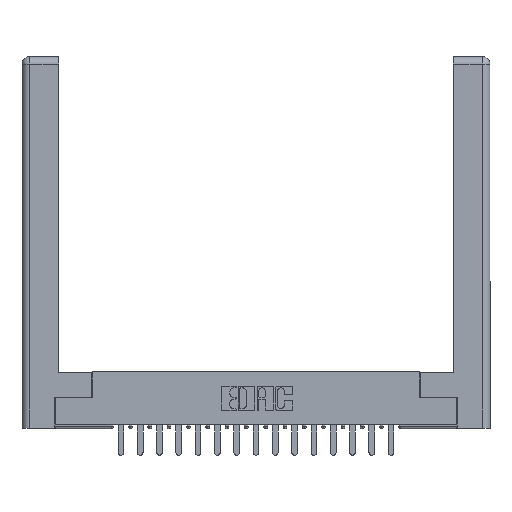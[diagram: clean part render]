
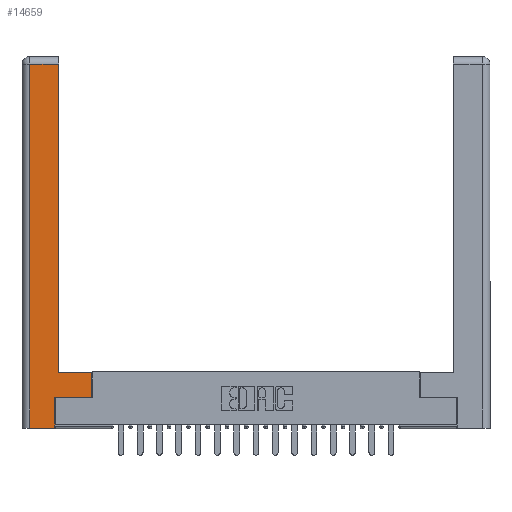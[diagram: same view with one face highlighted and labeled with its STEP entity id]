
A CAD part, top view. The second image highlights one B-rep face of the part: STEP entity #14659.
In plain terms, the highlighted planar face has unit normal (0, 0, 1).
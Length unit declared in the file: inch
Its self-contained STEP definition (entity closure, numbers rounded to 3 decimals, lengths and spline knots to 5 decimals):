
#138 = LINE ( 'NONE', #17752, #3976 ) ;
#511 = EDGE_CURVE ( 'NONE', #17838, #16991, #8730, .T. ) ;
#798 = ORIENTED_EDGE ( 'NONE', *, *, #15813, .T. ) ;
#850 = LINE ( 'NONE', #16740, #11092 ) ;
#1179 = CARTESIAN_POINT ( 'NONE',  ( 0.265, 0.245, 0. ) ) ;
#1506 = CARTESIAN_POINT ( 'NONE',  ( 0.0615, 2.94, 0. ) ) ;
#2007 = CARTESIAN_POINT ( 'NONE',  ( 0.0615, 2.94, 0. ) ) ;
#2164 = ORIENTED_EDGE ( 'NONE', *, *, #18892, .T. ) ;
#2183 = DIRECTION ( 'NONE',  ( 1., 0., 0. ) ) ;
#2369 = VECTOR ( 'NONE', #8172, 39.37008 ) ;
#2411 = FACE_OUTER_BOUND ( 'NONE', #13068, .T. ) ;
#2498 = EDGE_CURVE ( 'NONE', #12459, #17838, #14176, .T. ) ;
#2706 = PLANE ( 'NONE',  #8961 ) ;
#3361 = CARTESIAN_POINT ( 'NONE',  ( 0.565, 0.245, 0. ) ) ;
#3501 = VERTEX_POINT ( 'NONE', #12712 ) ;
#3976 = VECTOR ( 'NONE', #19290, 39.37008 ) ;
#4780 = CARTESIAN_POINT ( 'NONE',  ( 0.295, 0.45, 0. ) ) ;
#5429 = CARTESIAN_POINT ( 'NONE',  ( 0.295, 2.94, 0. ) ) ;
#5454 = ORIENTED_EDGE ( 'NONE', *, *, #511, .T. ) ;
#5558 = LINE ( 'NONE', #10978, #12875 ) ;
#5668 = EDGE_CURVE ( 'NONE', #6806, #17749, #12123, .T. ) ;
#6457 = DIRECTION ( 'NONE',  ( 0., -1., 0. ) ) ;
#6792 = DIRECTION ( 'NONE',  ( -1., 0., 0. ) ) ;
#6806 = VERTEX_POINT ( 'NONE', #5429 ) ;
#7336 = EDGE_CURVE ( 'NONE', #16514, #3501, #850, .T. ) ;
#7434 = DIRECTION ( 'NONE',  ( 0., 1., 0. ) ) ;
#8172 = DIRECTION ( 'NONE',  ( 0., 1., 0. ) ) ;
#8730 = LINE ( 'NONE', #9807, #2369 ) ;
#8961 = AXIS2_PLACEMENT_3D ( 'NONE', #15368, #13759, #16874 ) ;
#9242 = CARTESIAN_POINT ( 'NONE',  ( 0.295, 0.45, 0. ) ) ;
#9628 = ORIENTED_EDGE ( 'NONE', *, *, #2498, .T. ) ;
#9807 = CARTESIAN_POINT ( 'NONE',  ( 0.265, 0.245, 0. ) ) ;
#10978 = CARTESIAN_POINT ( 'NONE',  ( 0.0615, 0., 0. ) ) ;
#11092 = VECTOR ( 'NONE', #7434, 39.37008 ) ;
#11752 = EDGE_CURVE ( 'NONE', #3501, #14132, #11788, .T. ) ;
#11788 = LINE ( 'NONE', #9242, #13012 ) ;
#12063 = ORIENTED_EDGE ( 'NONE', *, *, #11752, .T. ) ;
#12123 = LINE ( 'NONE', #2007, #17464 ) ;
#12246 = ORIENTED_EDGE ( 'NONE', *, *, #5668, .T. ) ;
#12459 = VERTEX_POINT ( 'NONE', #13750 ) ;
#12528 = VECTOR ( 'NONE', #18963, 39.37008 ) ;
#12712 = CARTESIAN_POINT ( 'NONE',  ( 0.565, 0.45, 0. ) ) ;
#12875 = VECTOR ( 'NONE', #6457, 39.37008 ) ;
#13010 = LINE ( 'NONE', #3361, #12528 ) ;
#13012 = VECTOR ( 'NONE', #14075, 39.37008 ) ;
#13068 = EDGE_LOOP ( 'NONE', ( #2164, #12246, #798, #9628, #5454, #16052, #14321, #12063 ) ) ;
#13750 = CARTESIAN_POINT ( 'NONE',  ( 0.0615, 0., 0. ) ) ;
#13759 = DIRECTION ( 'NONE',  ( 0., 0., -1. ) ) ;
#14075 = DIRECTION ( 'NONE',  ( -1., 0., 0. ) ) ;
#14132 = VERTEX_POINT ( 'NONE', #4780 ) ;
#14176 = LINE ( 'NONE', #16131, #17561 ) ;
#14321 = ORIENTED_EDGE ( 'NONE', *, *, #7336, .T. ) ;
#14659 = ADVANCED_FACE ( 'NONE', ( #2411 ), #2706, .F. ) ;
#15368 = CARTESIAN_POINT ( 'NONE',  ( 0., 0., 0. ) ) ;
#15813 = EDGE_CURVE ( 'NONE', #17749, #12459, #5558, .T. ) ;
#16052 = ORIENTED_EDGE ( 'NONE', *, *, #18788, .T. ) ;
#16131 = CARTESIAN_POINT ( 'NONE',  ( 0.265, 0., 0. ) ) ;
#16514 = VERTEX_POINT ( 'NONE', #17511 ) ;
#16740 = CARTESIAN_POINT ( 'NONE',  ( 0.565, 0.45, 0. ) ) ;
#16874 = DIRECTION ( 'NONE',  ( -1., 0., 0. ) ) ;
#16991 = VERTEX_POINT ( 'NONE', #1179 ) ;
#17464 = VECTOR ( 'NONE', #6792, 39.37008 ) ;
#17511 = CARTESIAN_POINT ( 'NONE',  ( 0.565, 0.245, 0. ) ) ;
#17561 = VECTOR ( 'NONE', #2183, 39.37008 ) ;
#17749 = VERTEX_POINT ( 'NONE', #1506 ) ;
#17752 = CARTESIAN_POINT ( 'NONE',  ( 0.295, 3., 0. ) ) ;
#17838 = VERTEX_POINT ( 'NONE', #19398 ) ;
#18788 = EDGE_CURVE ( 'NONE', #16991, #16514, #13010, .T. ) ;
#18892 = EDGE_CURVE ( 'NONE', #14132, #6806, #138, .T. ) ;
#18963 = DIRECTION ( 'NONE',  ( 1., 0., 0. ) ) ;
#19290 = DIRECTION ( 'NONE',  ( 0., 1., 0. ) ) ;
#19398 = CARTESIAN_POINT ( 'NONE',  ( 0.265, 0., 0. ) ) ;
